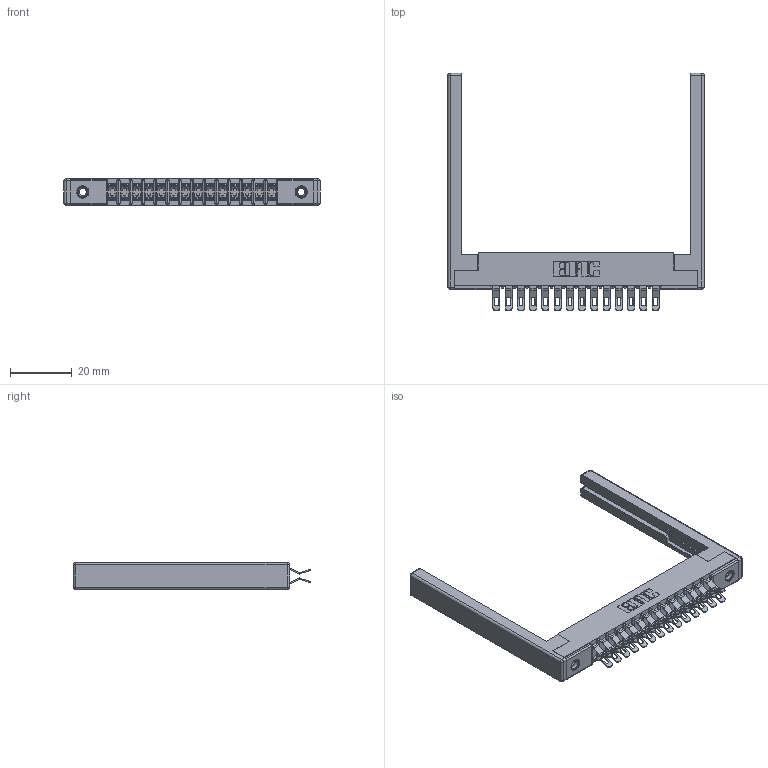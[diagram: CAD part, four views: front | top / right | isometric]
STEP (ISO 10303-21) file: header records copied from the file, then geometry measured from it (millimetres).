
FILE_DESCRIPTION (( 'STEP AP203' ), '1' );
FILE_NAME ('307-028-555-268.STEP', '2019-09-05T23:59:04', ( '' ), ( '' ), 'SwSTEP 2.0', 'SolidWorks 2016', '' );
FILE_SCHEMA (( 'CONFIG_CONTROL_DESIGN' ));
Length unit declared in the file: inch
Products named in the file (5): 307 Part_.156 Dia Mounting Holes; 345-250-001_345-250-001-102; 307-290-001_555; 307-028-555-268; 307-220-068
Assembly tree (33 placements, depth 2):
  307-028-555-268
    307 Part_.156 Dia Mounting Holes
    307-290-001_555  x28
    307-220-068  x2
    345-250-001_345-250-001-102  x2
Bounding box: 82.91 x 76.71 x 8.71 mm (x, y, z)
Volume: 10068.7 mm3; surface area: 13814.6 mm2
Topology: 33 solids, 33 shells, 1995 faces, 5781 edges, 3754 vertices
Faces by surface type: plane 1110, cylinder 831, sphere 38, cone 12, torus 4
Entity records: 19198 total; most frequent: CARTESIAN_POINT 3131, DIRECTION 3101, ORIENTED_EDGE 3094, EDGE_CURVE 1547, LINE 1161, VECTOR 1161, VERTEX_POINT 1000, AXIS2_PLACEMENT_3D 970
